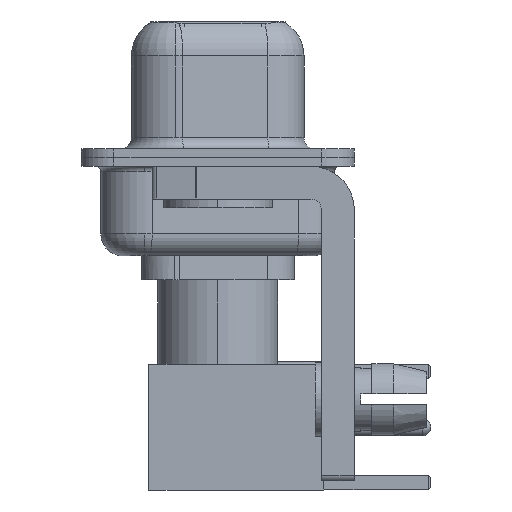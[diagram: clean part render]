
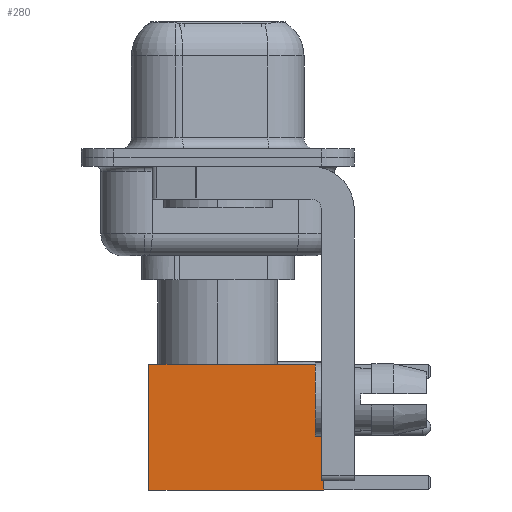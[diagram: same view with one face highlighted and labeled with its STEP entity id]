
A CAD part, left-side view. The second image highlights one B-rep face of the part: STEP entity #280.
In plain terms, the highlighted face is planar.
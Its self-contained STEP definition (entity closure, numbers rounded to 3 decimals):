
#280 = ADVANCED_FACE ( 'NONE', ( #10569 ), #1632, .T. ) ;
#1062 = LINE ( 'NONE', #4873, #11332 ) ;
#1632 = PLANE ( 'NONE',  #2404 ) ;
#1746 = CARTESIAN_POINT ( 'NONE',  ( 2.875, 2.875, 0. ) ) ;
#1760 = DIRECTION ( 'NONE',  ( 0., 1., 0. ) ) ;
#1833 = LINE ( 'NONE', #5282, #5637 ) ;
#1928 = ORIENTED_EDGE ( 'NONE', *, *, #15544, .T. ) ;
#2404 = AXIS2_PLACEMENT_3D ( 'NONE', #23374, #1760, #17745 ) ;
#3178 = ORIENTED_EDGE ( 'NONE', *, *, #21050, .F. ) ;
#3778 = ORIENTED_EDGE ( 'NONE', *, *, #17837, .T. ) ;
#3855 = DIRECTION ( 'NONE',  ( 0., 0., -1. ) ) ;
#3985 = DIRECTION ( 'NONE',  ( 0., 0., -1. ) ) ;
#4416 = VERTEX_POINT ( 'NONE', #16515 ) ;
#4676 = CARTESIAN_POINT ( 'NONE',  ( -2.875, 2.875, 0. ) ) ;
#4873 = CARTESIAN_POINT ( 'NONE',  ( 0., 2.875, 0. ) ) ;
#5188 = LINE ( 'NONE', #18867, #16740 ) ;
#5282 = CARTESIAN_POINT ( 'NONE',  ( 2.875, 2.875, 0. ) ) ;
#5637 = VECTOR ( 'NONE', #3855, 1000. ) ;
#6140 = VECTOR ( 'NONE', #3985, 1000. ) ;
#6336 = DIRECTION ( 'NONE',  ( -1., 0., 0. ) ) ;
#7995 = EDGE_CURVE ( 'NONE', #9774, #9624, #16854, .T. ) ;
#9560 = CARTESIAN_POINT ( 'NONE',  ( -2.875, 2.875, 0. ) ) ;
#9624 = VERTEX_POINT ( 'NONE', #4676 ) ;
#9774 = VERTEX_POINT ( 'NONE', #22741 ) ;
#10346 = DIRECTION ( 'NONE',  ( -1., 0., 0. ) ) ;
#10569 = FACE_OUTER_BOUND ( 'NONE', #17096, .T. ) ;
#11332 = VECTOR ( 'NONE', #10346, 1000. ) ;
#12364 = ORIENTED_EDGE ( 'NONE', *, *, #7995, .F. ) ;
#15544 = EDGE_CURVE ( 'NONE', #4416, #22470, #1833, .T. ) ;
#16515 = CARTESIAN_POINT ( 'NONE',  ( 2.875, 2.875, 8. ) ) ;
#16740 = VECTOR ( 'NONE', #6336, 1000. ) ;
#16854 = LINE ( 'NONE', #9560, #6140 ) ;
#17096 = EDGE_LOOP ( 'NONE', ( #1928, #3778, #12364, #3178 ) ) ;
#17745 = DIRECTION ( 'NONE',  ( 0., 0., 1. ) ) ;
#17837 = EDGE_CURVE ( 'NONE', #22470, #9624, #1062, .T. ) ;
#18867 = CARTESIAN_POINT ( 'NONE',  ( 0., 2.875, 8. ) ) ;
#21050 = EDGE_CURVE ( 'NONE', #4416, #9774, #5188, .T. ) ;
#22470 = VERTEX_POINT ( 'NONE', #1746 ) ;
#22741 = CARTESIAN_POINT ( 'NONE',  ( -2.875, 2.875, 8. ) ) ;
#23374 = CARTESIAN_POINT ( 'NONE',  ( 2.875, 2.875, 0. ) ) ;
